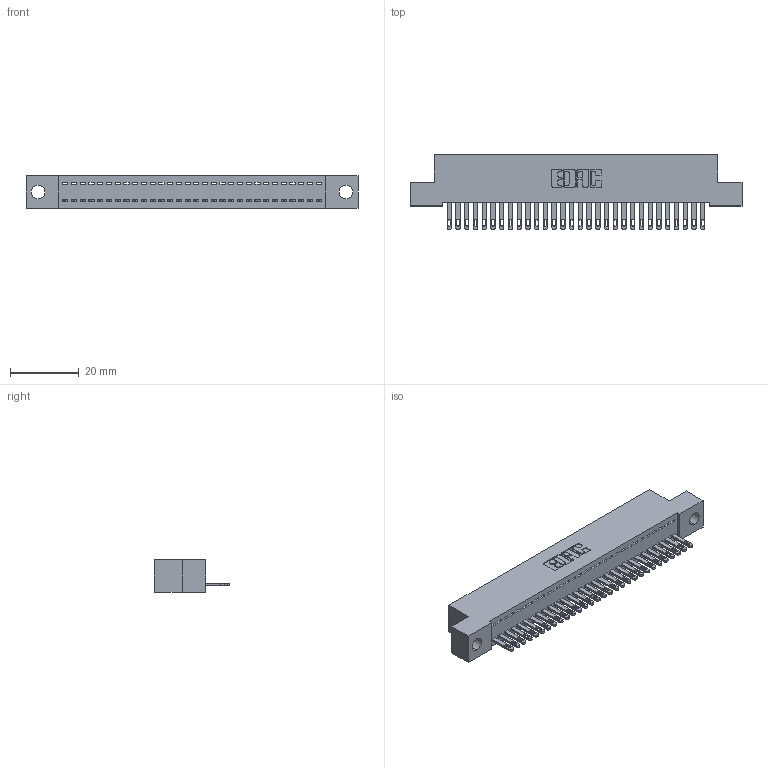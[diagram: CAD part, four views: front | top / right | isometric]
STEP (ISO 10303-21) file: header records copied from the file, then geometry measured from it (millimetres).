
FILE_DESCRIPTION (( 'STEP AP203' ), '1' );
FILE_NAME ('892-030-500-104.STEP', '2020-09-21T15:05:47', ( '' ), ( '' ), 'SwSTEP 2.0', 'SolidWorks 2020', '' );
FILE_SCHEMA (( 'CONFIG_CONTROL_DESIGN' ));
Length unit declared in the file: inch
Products named in the file (3): 345-292-001_345-293-100; 842 Part_.156 TH; 892-030-500-104
Assembly tree (31 placements, depth 2):
  892-030-500-104
    842 Part_.156 TH
    345-292-001_345-293-100  x30
Bounding box: 96.52 x 21.85 x 9.4 mm (x, y, z)
Volume: 8350.2 mm3; surface area: 11915.7 mm2
Topology: 31 solids, 31 shells, 1730 faces, 5339 edges, 3558 vertices
Faces by surface type: plane 1146, cylinder 584
Entity records: 19693 total; most frequent: CARTESIAN_POINT 3404, ORIENTED_EDGE 3370, DIRECTION 2897, EDGE_CURVE 1685, LINE 1553, VECTOR 1553, VERTEX_POINT 1122, AXIS2_PLACEMENT_3D 672
